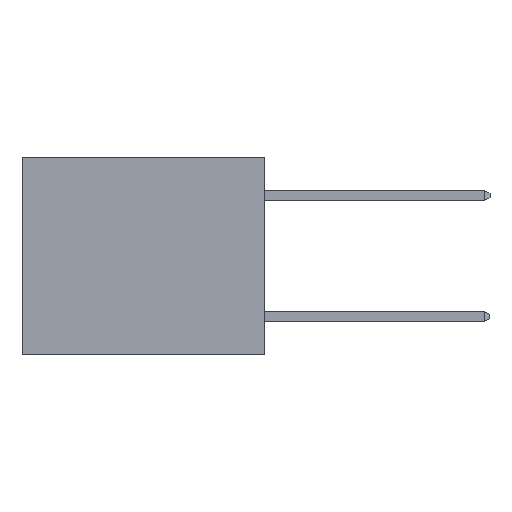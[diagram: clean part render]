
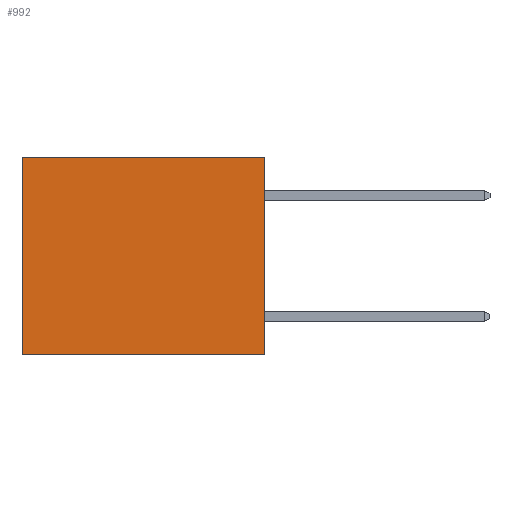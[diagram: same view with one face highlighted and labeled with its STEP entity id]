
A CAD part, left-side view. The second image highlights one B-rep face of the part: STEP entity #992.
In plain terms, the highlighted planar face has unit normal (-1, 0, 0).
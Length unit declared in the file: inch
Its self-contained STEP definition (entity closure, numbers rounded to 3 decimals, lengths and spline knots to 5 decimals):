
#2 = DIRECTION ( 'NONE',  ( 0., 0., -1. ) ) ;
#78 = VERTEX_POINT ( 'NONE', #4266 ) ;
#285 = CARTESIAN_POINT ( 'NONE',  ( 0.3165, 0., -0.49 ) ) ;
#309 = DIRECTION ( 'NONE',  ( 0., 1., 0. ) ) ;
#349 = EDGE_CURVE ( 'NONE', #7760, #78, #3272, .T. ) ;
#461 = CARTESIAN_POINT ( 'NONE',  ( 0.3165, 0., 0. ) ) ;
#815 = EDGE_CURVE ( 'NONE', #7760, #6711, #4180, .T. ) ;
#992 = ADVANCED_FACE ( 'NONE', ( #8185 ), #2820, .F. ) ;
#1467 = CARTESIAN_POINT ( 'NONE',  ( 0.3165, 0., -0.49 ) ) ;
#2095 = CARTESIAN_POINT ( 'NONE',  ( 0.3165, 0., -0.49 ) ) ;
#2223 = CARTESIAN_POINT ( 'NONE',  ( 0.3165, 0.6, -0.49 ) ) ;
#2597 = ORIENTED_EDGE ( 'NONE', *, *, #349, .F. ) ;
#2603 = VECTOR ( 'NONE', #309, 39.37008 ) ;
#2820 = PLANE ( 'NONE',  #3365 ) ;
#3075 = LINE ( 'NONE', #5979, #6410 ) ;
#3248 = EDGE_CURVE ( 'NONE', #78, #7618, #4291, .T. ) ;
#3272 = LINE ( 'NONE', #1467, #3374 ) ;
#3365 = AXIS2_PLACEMENT_3D ( 'NONE', #2095, #6605, #4050 ) ;
#3374 = VECTOR ( 'NONE', #3409, 39.37008 ) ;
#3409 = DIRECTION ( 'NONE',  ( 0., 0., -1. ) ) ;
#3448 = DIRECTION ( 'NONE',  ( 0., 1., 0. ) ) ;
#3776 = EDGE_LOOP ( 'NONE', ( #6917, #4928, #2597, #4092 ) ) ;
#4050 = DIRECTION ( 'NONE',  ( 0., 0., -1. ) ) ;
#4092 = ORIENTED_EDGE ( 'NONE', *, *, #815, .T. ) ;
#4175 = EDGE_CURVE ( 'NONE', #6711, #7618, #3075, .T. ) ;
#4180 = LINE ( 'NONE', #6660, #6291 ) ;
#4266 = CARTESIAN_POINT ( 'NONE',  ( 0.3165, 0., -0.49 ) ) ;
#4291 = LINE ( 'NONE', #285, #2603 ) ;
#4709 = CARTESIAN_POINT ( 'NONE',  ( 0.3165, 0.6, 0. ) ) ;
#4928 = ORIENTED_EDGE ( 'NONE', *, *, #3248, .F. ) ;
#5979 = CARTESIAN_POINT ( 'NONE',  ( 0.3165, 0.6, -0.49 ) ) ;
#6291 = VECTOR ( 'NONE', #3448, 39.37008 ) ;
#6410 = VECTOR ( 'NONE', #2, 39.37008 ) ;
#6605 = DIRECTION ( 'NONE',  ( 1., 0., 0. ) ) ;
#6660 = CARTESIAN_POINT ( 'NONE',  ( 0.3165, 0., 0. ) ) ;
#6711 = VERTEX_POINT ( 'NONE', #4709 ) ;
#6917 = ORIENTED_EDGE ( 'NONE', *, *, #4175, .T. ) ;
#7618 = VERTEX_POINT ( 'NONE', #2223 ) ;
#7760 = VERTEX_POINT ( 'NONE', #461 ) ;
#8185 = FACE_OUTER_BOUND ( 'NONE', #3776, .T. ) ;
